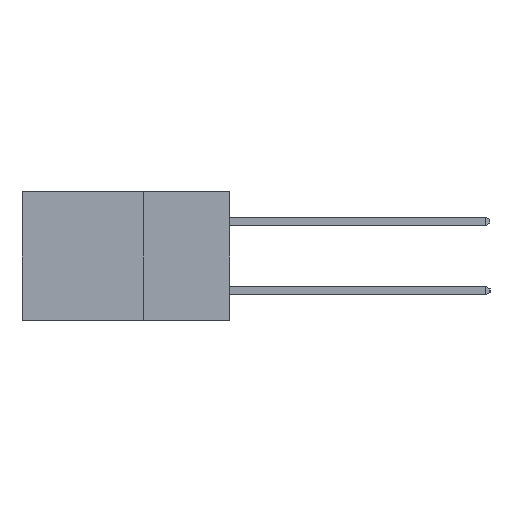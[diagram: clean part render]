
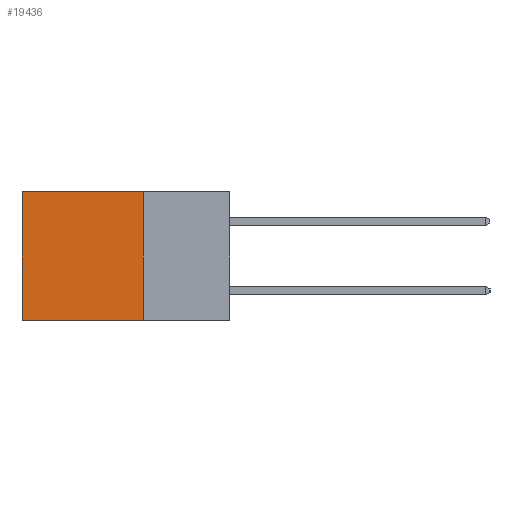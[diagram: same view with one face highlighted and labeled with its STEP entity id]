
A CAD part, left-side view. The second image highlights one B-rep face of the part: STEP entity #19436.
In plain terms, the highlighted planar face has unit normal (-1, 0, 0).
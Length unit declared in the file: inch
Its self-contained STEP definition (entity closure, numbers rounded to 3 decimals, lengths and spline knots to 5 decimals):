
#679 = DIRECTION ( 'NONE',  ( 0., 0., -1. ) ) ;
#1156 = VECTOR ( 'NONE', #12457, 39.37008 ) ;
#2143 = VERTEX_POINT ( 'NONE', #3737 ) ;
#2400 = CARTESIAN_POINT ( 'NONE',  ( 0.2615, 0.6, 0. ) ) ;
#3014 = CARTESIAN_POINT ( 'NONE',  ( 0.2615, 0.6, -0.37 ) ) ;
#3737 = CARTESIAN_POINT ( 'NONE',  ( 0.2615, 0.25, 0. ) ) ;
#3768 = EDGE_CURVE ( 'NONE', #16692, #17102, #11832, .T. ) ;
#3805 = DIRECTION ( 'NONE',  ( 0., 1., 0. ) ) ;
#4344 = AXIS2_PLACEMENT_3D ( 'NONE', #5741, #10828, #679 ) ;
#4830 = ORIENTED_EDGE ( 'NONE', *, *, #3768, .F. ) ;
#5045 = ORIENTED_EDGE ( 'NONE', *, *, #10746, .F. ) ;
#5661 = LINE ( 'NONE', #5713, #1156 ) ;
#5713 = CARTESIAN_POINT ( 'NONE',  ( 0.2615, 0.25, -0.37 ) ) ;
#5741 = CARTESIAN_POINT ( 'NONE',  ( 0.2615, 0.25, -0.37 ) ) ;
#6569 = ORIENTED_EDGE ( 'NONE', *, *, #21183, .T. ) ;
#6821 = EDGE_CURVE ( 'NONE', #20141, #17102, #16862, .T. ) ;
#8010 = VECTOR ( 'NONE', #18794, 39.37008 ) ;
#8100 = FACE_OUTER_BOUND ( 'NONE', #9619, .T. ) ;
#8559 = LINE ( 'NONE', #17091, #8010 ) ;
#9619 = EDGE_LOOP ( 'NONE', ( #9644, #4830, #5045, #6569 ) ) ;
#9644 = ORIENTED_EDGE ( 'NONE', *, *, #6821, .T. ) ;
#10746 = EDGE_CURVE ( 'NONE', #2143, #16692, #5661, .T. ) ;
#10828 = DIRECTION ( 'NONE',  ( 1., 0., 0. ) ) ;
#11832 = LINE ( 'NONE', #16857, #21359 ) ;
#12169 = CARTESIAN_POINT ( 'NONE',  ( 0.2615, 0.25, -0.37 ) ) ;
#12457 = DIRECTION ( 'NONE',  ( 0., 0., -1. ) ) ;
#13200 = CARTESIAN_POINT ( 'NONE',  ( 0.2615, 0.6, -0.37 ) ) ;
#13204 = DIRECTION ( 'NONE',  ( 0., 0., -1. ) ) ;
#16692 = VERTEX_POINT ( 'NONE', #12169 ) ;
#16857 = CARTESIAN_POINT ( 'NONE',  ( 0.2615, 0.25, -0.37 ) ) ;
#16862 = LINE ( 'NONE', #13200, #21390 ) ;
#17091 = CARTESIAN_POINT ( 'NONE',  ( 0.2615, 0.25, 0. ) ) ;
#17102 = VERTEX_POINT ( 'NONE', #3014 ) ;
#18794 = DIRECTION ( 'NONE',  ( 0., 1., 0. ) ) ;
#19436 = ADVANCED_FACE ( 'NONE', ( #8100 ), #20947, .F. ) ;
#20141 = VERTEX_POINT ( 'NONE', #2400 ) ;
#20947 = PLANE ( 'NONE',  #4344 ) ;
#21183 = EDGE_CURVE ( 'NONE', #2143, #20141, #8559, .T. ) ;
#21359 = VECTOR ( 'NONE', #3805, 39.37008 ) ;
#21390 = VECTOR ( 'NONE', #13204, 39.37008 ) ;
